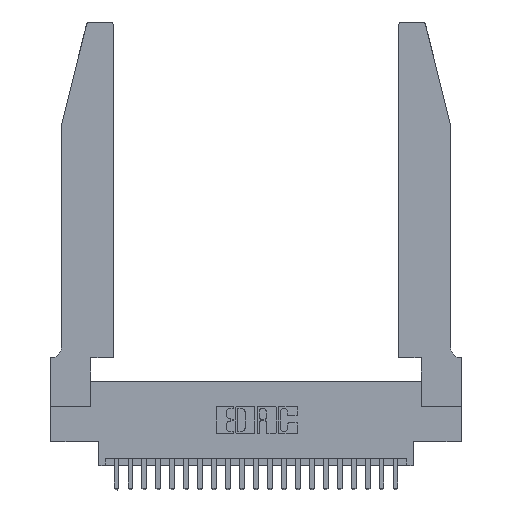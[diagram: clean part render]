
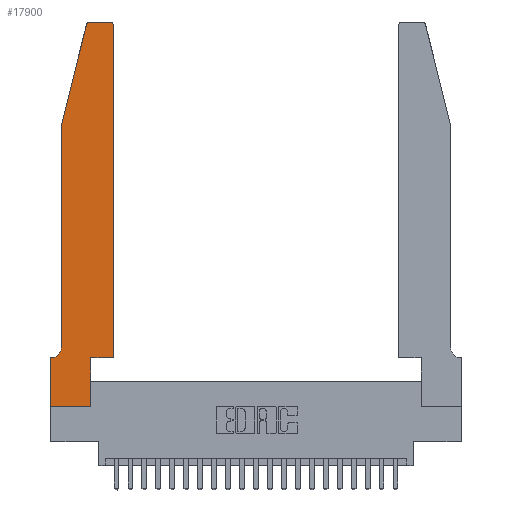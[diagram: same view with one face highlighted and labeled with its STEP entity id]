
A CAD part, top view. The second image highlights one B-rep face of the part: STEP entity #17900.
In plain terms, the highlighted planar face has unit normal (0, 0, 1).
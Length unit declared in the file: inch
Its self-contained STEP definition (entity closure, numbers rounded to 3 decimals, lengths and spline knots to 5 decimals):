
#667 = DIRECTION ( 'NONE',  ( 0., 0., 1. ) ) ;
#763 = ORIENTED_EDGE ( 'NONE', *, *, #17582, .T. ) ;
#876 = VECTOR ( 'NONE', #6098, 39.37008 ) ;
#1488 = VERTEX_POINT ( 'NONE', #13773 ) ;
#1511 = EDGE_CURVE ( 'NONE', #6314, #13647, #16643, .T. ) ;
#1542 = CARTESIAN_POINT ( 'NONE',  ( 0., 0.35, 0.37 ) ) ;
#1908 = CIRCLE ( 'NONE', #24086, 0.03 ) ;
#2234 = EDGE_CURVE ( 'NONE', #24108, #6314, #18089, .T. ) ;
#2316 = ORIENTED_EDGE ( 'NONE', *, *, #20721, .T. ) ;
#3178 = CARTESIAN_POINT ( 'NONE',  ( 0.0755, 0.42, 0.37 ) ) ;
#3302 = VERTEX_POINT ( 'NONE', #3871 ) ;
#3761 = LINE ( 'NONE', #15529, #23158 ) ;
#3871 = CARTESIAN_POINT ( 'NONE',  ( 0.0755, 2., 0.37 ) ) ;
#3979 = DIRECTION ( 'NONE',  ( -0.239, -0.971, 0. ) ) ;
#4316 = VECTOR ( 'NONE', #17459, 39.37008 ) ;
#4322 = EDGE_CURVE ( 'NONE', #18956, #24108, #11201, .T. ) ;
#4574 = DIRECTION ( 'NONE',  ( 1., 0., 0. ) ) ;
#4590 = CARTESIAN_POINT ( 'NONE',  ( 0.2865, 0., 0.37 ) ) ;
#4632 = VERTEX_POINT ( 'NONE', #20238 ) ;
#5043 = VERTEX_POINT ( 'NONE', #15595 ) ;
#5309 = DIRECTION ( 'NONE',  ( 0., 1., 0. ) ) ;
#6098 = DIRECTION ( 'NONE',  ( -1., 0., 0. ) ) ;
#6220 = VECTOR ( 'NONE', #10683, 39.37008 ) ;
#6314 = VERTEX_POINT ( 'NONE', #18042 ) ;
#6340 = VECTOR ( 'NONE', #18821, 39.37008 ) ;
#6372 = CARTESIAN_POINT ( 'NONE',  ( 0.2865, 0.35, 0.37 ) ) ;
#6820 = CARTESIAN_POINT ( 'NONE',  ( 0.4505, 0.35, 0.37 ) ) ;
#7014 = CARTESIAN_POINT ( 'NONE',  ( 0.0755, 0.35, 0.37 ) ) ;
#7190 = CARTESIAN_POINT ( 'NONE',  ( 0.4505, 0.35, 0.37 ) ) ;
#7731 = CARTESIAN_POINT ( 'NONE',  ( 0., 0., 0.37 ) ) ;
#7732 = VECTOR ( 'NONE', #12908, 39.37008 ) ;
#8038 = VERTEX_POINT ( 'NONE', #6372 ) ;
#8042 = DIRECTION ( 'NONE',  ( 0., -1., 0. ) ) ;
#8454 = ORIENTED_EDGE ( 'NONE', *, *, #20729, .T. ) ;
#8755 = DIRECTION ( 'NONE',  ( 0., 0., -1. ) ) ;
#8825 = DIRECTION ( 'NONE',  ( 1., 0., 0. ) ) ;
#8958 = ORIENTED_EDGE ( 'NONE', *, *, #1511, .T. ) ;
#9778 = AXIS2_PLACEMENT_3D ( 'NONE', #21245, #667, #14306 ) ;
#10133 = EDGE_CURVE ( 'NONE', #14710, #18904, #1908, .T. ) ;
#10240 = CARTESIAN_POINT ( 'NONE',  ( 0., 0.35, 0.37 ) ) ;
#10683 = DIRECTION ( 'NONE',  ( -1., 0., 0. ) ) ;
#10787 = EDGE_CURVE ( 'NONE', #5043, #3302, #11508, .T. ) ;
#10864 = EDGE_CURVE ( 'NONE', #13328, #18956, #21242, .T. ) ;
#11200 = ORIENTED_EDGE ( 'NONE', *, *, #21028, .T. ) ;
#11201 = LINE ( 'NONE', #7014, #6220 ) ;
#11508 = LINE ( 'NONE', #21027, #20324 ) ;
#11866 = CARTESIAN_POINT ( 'NONE',  ( 0.2865, 0.35, 0.37 ) ) ;
#12116 = LINE ( 'NONE', #7190, #7732 ) ;
#12507 = CARTESIAN_POINT ( 'NONE',  ( 0.4505, 2.72, 0.37 ) ) ;
#12756 = CIRCLE ( 'NONE', #9778, 0.03 ) ;
#12802 = EDGE_CURVE ( 'NONE', #4632, #5043, #12756, .T. ) ;
#12908 = DIRECTION ( 'NONE',  ( 1., 0., 0. ) ) ;
#12940 = ORIENTED_EDGE ( 'NONE', *, *, #10787, .T. ) ;
#13086 = ORIENTED_EDGE ( 'NONE', *, *, #13874, .T. ) ;
#13328 = VERTEX_POINT ( 'NONE', #3178 ) ;
#13647 = VERTEX_POINT ( 'NONE', #4590 ) ;
#13773 = CARTESIAN_POINT ( 'NONE',  ( 0.4505, 0.35, 0.37 ) ) ;
#13874 = EDGE_CURVE ( 'NONE', #8038, #1488, #12116, .T. ) ;
#13906 = CARTESIAN_POINT ( 'NONE',  ( 0.4205, 2.72, 0.37 ) ) ;
#14006 = CARTESIAN_POINT ( 'NONE',  ( 0.4205, 2.75, 0.37 ) ) ;
#14306 = DIRECTION ( 'NONE',  ( 1., 0., 0. ) ) ;
#14526 = ORIENTED_EDGE ( 'NONE', *, *, #10864, .T. ) ;
#14597 = ORIENTED_EDGE ( 'NONE', *, *, #10133, .T. ) ;
#14710 = VERTEX_POINT ( 'NONE', #12507 ) ;
#15135 = ORIENTED_EDGE ( 'NONE', *, *, #12802, .T. ) ;
#15410 = VECTOR ( 'NONE', #19441, 39.37008 ) ;
#15450 = CARTESIAN_POINT ( 'NONE',  ( 0., 0., 0.37 ) ) ;
#15529 = CARTESIAN_POINT ( 'NONE',  ( 0.0755, 2., 0.37 ) ) ;
#15595 = CARTESIAN_POINT ( 'NONE',  ( 0.25487, 2.72718, 0.37 ) ) ;
#16416 = ORIENTED_EDGE ( 'NONE', *, *, #4322, .T. ) ;
#16643 = LINE ( 'NONE', #15450, #15410 ) ;
#16664 = FACE_OUTER_BOUND ( 'NONE', #17801, .T. ) ;
#16690 = CARTESIAN_POINT ( 'NONE',  ( 0.0055, 0.42, 0.37 ) ) ;
#17270 = AXIS2_PLACEMENT_3D ( 'NONE', #16690, #8755, #23718 ) ;
#17459 = DIRECTION ( 'NONE',  ( 0., 1., 0. ) ) ;
#17582 = EDGE_CURVE ( 'NONE', #18904, #4632, #19619, .T. ) ;
#17801 = EDGE_LOOP ( 'NONE', ( #763, #15135, #12940, #8454, #14526, #16416, #20785, #8958, #2316, #13086, #11200, #14597 ) ) ;
#17900 = ADVANCED_FACE ( 'NONE', ( #16664 ), #20044, .T. ) ;
#18042 = CARTESIAN_POINT ( 'NONE',  ( 0., 0., 0.37 ) ) ;
#18089 = LINE ( 'NONE', #7731, #6340 ) ;
#18103 = VECTOR ( 'NONE', #5309, 39.37008 ) ;
#18821 = DIRECTION ( 'NONE',  ( 0., -1., 0. ) ) ;
#18904 = VERTEX_POINT ( 'NONE', #14006 ) ;
#18956 = VERTEX_POINT ( 'NONE', #19844 ) ;
#19284 = LINE ( 'NONE', #11866, #4316 ) ;
#19420 = DIRECTION ( 'NONE',  ( 0., 0., 1. ) ) ;
#19441 = DIRECTION ( 'NONE',  ( 1., 0., 0. ) ) ;
#19619 = LINE ( 'NONE', #20795, #876 ) ;
#19844 = CARTESIAN_POINT ( 'NONE',  ( 0.0055, 0.35, 0.37 ) ) ;
#20044 = PLANE ( 'NONE',  #20384 ) ;
#20238 = CARTESIAN_POINT ( 'NONE',  ( 0.284, 2.75, 0.37 ) ) ;
#20324 = VECTOR ( 'NONE', #3979, 39.37008 ) ;
#20384 = AXIS2_PLACEMENT_3D ( 'NONE', #1542, #21941, #8825 ) ;
#20721 = EDGE_CURVE ( 'NONE', #13647, #8038, #19284, .T. ) ;
#20729 = EDGE_CURVE ( 'NONE', #3302, #13328, #3761, .T. ) ;
#20785 = ORIENTED_EDGE ( 'NONE', *, *, #2234, .T. ) ;
#20795 = CARTESIAN_POINT ( 'NONE',  ( 0.2605, 2.75, 0.37 ) ) ;
#21027 = CARTESIAN_POINT ( 'NONE',  ( 0.0755, 2., 0.37 ) ) ;
#21028 = EDGE_CURVE ( 'NONE', #1488, #14710, #24316, .T. ) ;
#21242 = CIRCLE ( 'NONE', #17270, 0.07 ) ;
#21245 = CARTESIAN_POINT ( 'NONE',  ( 0.284, 2.72, 0.37 ) ) ;
#21941 = DIRECTION ( 'NONE',  ( 0., 0., 1. ) ) ;
#23158 = VECTOR ( 'NONE', #8042, 39.37008 ) ;
#23718 = DIRECTION ( 'NONE',  ( -1., 0., 0. ) ) ;
#24086 = AXIS2_PLACEMENT_3D ( 'NONE', #13906, #19420, #4574 ) ;
#24108 = VERTEX_POINT ( 'NONE', #10240 ) ;
#24316 = LINE ( 'NONE', #6820, #18103 ) ;
